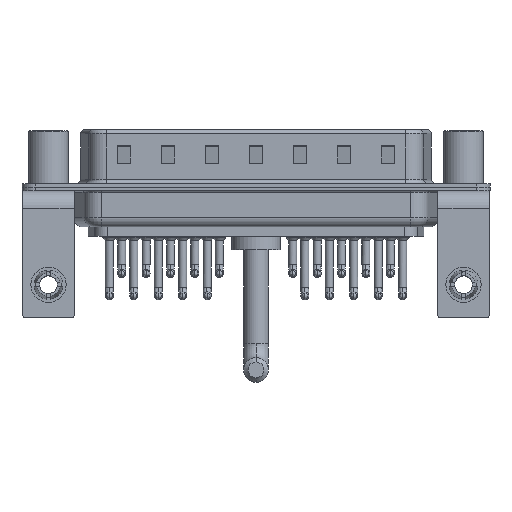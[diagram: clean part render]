
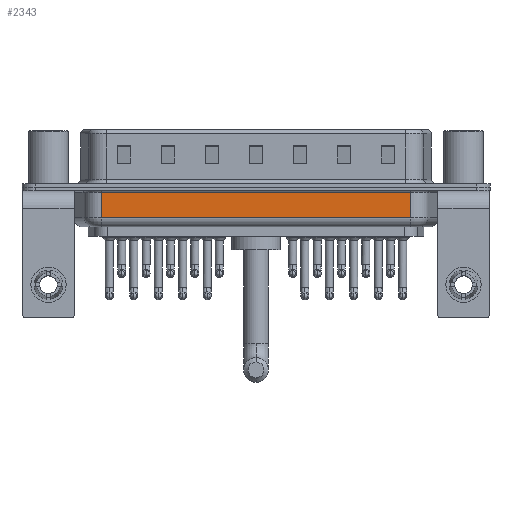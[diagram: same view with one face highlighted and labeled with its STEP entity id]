
A CAD part, front view. The second image highlights one B-rep face of the part: STEP entity #2343.
In plain terms, the highlighted planar face has unit normal (0, -1, 0).
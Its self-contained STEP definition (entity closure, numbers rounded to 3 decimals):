
#811 = CARTESIAN_POINT ( 'NONE',  ( 6.006, -5.35, -4.5 ) ) ;
#995 = AXIS2_PLACEMENT_3D ( 'NONE', #19873, #22404, #1698 ) ;
#1055 = CARTESIAN_POINT ( 'NONE',  ( 41.044, -5.35, -4.5 ) ) ;
#1698 = DIRECTION ( 'NONE',  ( 0., 0., 1. ) ) ;
#2343 = ADVANCED_FACE ( 'NONE', ( #10644 ), #6616, .F. ) ;
#2535 = LINE ( 'NONE', #9243, #16356 ) ;
#4510 = CARTESIAN_POINT ( 'NONE',  ( 6.006, -5.35, -3.5 ) ) ;
#5468 = VECTOR ( 'NONE', #9905, 1000. ) ;
#5985 = EDGE_CURVE ( 'NONE', #29134, #24478, #21233, .T. ) ;
#6273 = VERTEX_POINT ( 'NONE', #27983 ) ;
#6616 = PLANE ( 'NONE',  #995 ) ;
#9073 = ORIENTED_EDGE ( 'NONE', *, *, #14931, .T. ) ;
#9089 = DIRECTION ( 'NONE',  ( -1., 0., 0. ) ) ;
#9243 = CARTESIAN_POINT ( 'NONE',  ( 6.006, -5.35, -0.65 ) ) ;
#9640 = ORIENTED_EDGE ( 'NONE', *, *, #16293, .T. ) ;
#9905 = DIRECTION ( 'NONE',  ( 0., 0., 1. ) ) ;
#10559 = ORIENTED_EDGE ( 'NONE', *, *, #28317, .T. ) ;
#10644 = FACE_OUTER_BOUND ( 'NONE', #12235, .T. ) ;
#11570 = CARTESIAN_POINT ( 'NONE',  ( 6.006, -5.35, -0.65 ) ) ;
#12235 = EDGE_LOOP ( 'NONE', ( #18493, #10559, #9073, #9640 ) ) ;
#13571 = CARTESIAN_POINT ( 'NONE',  ( 41.044, -5.35, -3.5 ) ) ;
#14030 = LINE ( 'NONE', #4510, #22094 ) ;
#14546 = VERTEX_POINT ( 'NONE', #13571 ) ;
#14931 = EDGE_CURVE ( 'NONE', #14546, #6273, #22047, .T. ) ;
#16293 = EDGE_CURVE ( 'NONE', #6273, #24478, #2535, .T. ) ;
#16356 = VECTOR ( 'NONE', #9089, 1000. ) ;
#18493 = ORIENTED_EDGE ( 'NONE', *, *, #5985, .F. ) ;
#19873 = CARTESIAN_POINT ( 'NONE',  ( 6.006, -5.35, -4.5 ) ) ;
#21233 = LINE ( 'NONE', #811, #5468 ) ;
#22047 = LINE ( 'NONE', #1055, #23881 ) ;
#22094 = VECTOR ( 'NONE', #23113, 1000. ) ;
#22404 = DIRECTION ( 'NONE',  ( 0., 1., 0. ) ) ;
#23113 = DIRECTION ( 'NONE',  ( 1., 0., 0. ) ) ;
#23881 = VECTOR ( 'NONE', #28718, 1000. ) ;
#24478 = VERTEX_POINT ( 'NONE', #11570 ) ;
#24534 = CARTESIAN_POINT ( 'NONE',  ( 6.006, -5.35, -3.5 ) ) ;
#27983 = CARTESIAN_POINT ( 'NONE',  ( 41.044, -5.35, -0.65 ) ) ;
#28317 = EDGE_CURVE ( 'NONE', #29134, #14546, #14030, .T. ) ;
#28718 = DIRECTION ( 'NONE',  ( 0., 0., 1. ) ) ;
#29134 = VERTEX_POINT ( 'NONE', #24534 ) ;
